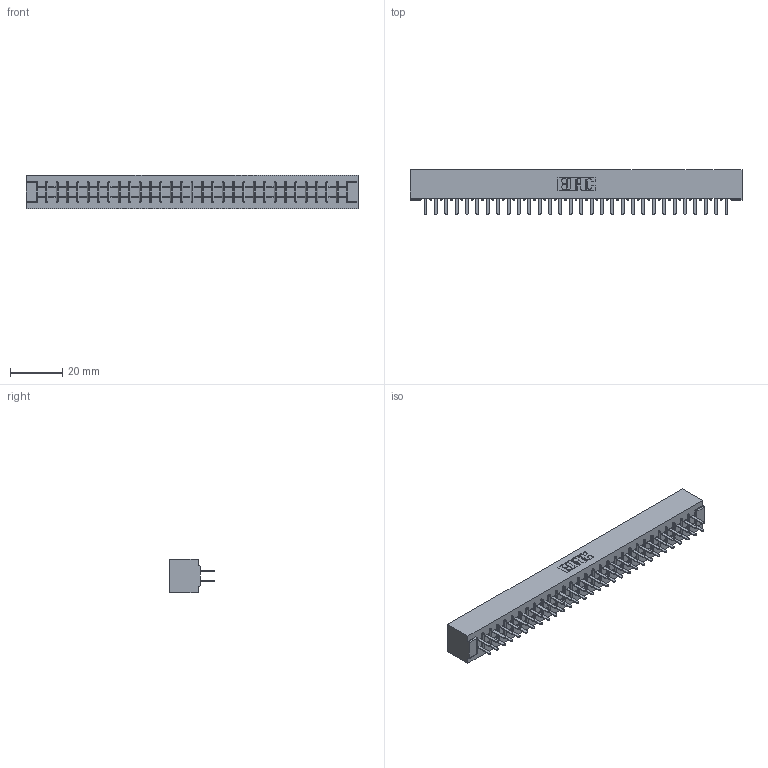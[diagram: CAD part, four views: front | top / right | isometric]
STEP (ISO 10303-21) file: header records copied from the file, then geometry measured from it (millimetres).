
FILE_DESCRIPTION (( 'STEP AP203' ), '1' );
FILE_NAME ('355-060-520-201.STEP', '2019-09-12T13:43:40', ( '' ), ( '' ), 'SwSTEP 2.0', 'SolidWorks 2016', '' );
FILE_SCHEMA (( 'CONFIG_CONTROL_DESIGN' ));
Length unit declared in the file: inch
Products named in the file (3): 355-060-520-201; 305-290-001_520; 305 Part_No Mounting
Assembly tree (61 placements, depth 2):
  355-060-520-201
    305 Part_No Mounting
    305-290-001_520  x60
Bounding box: 126.75 x 17.09 x 12.7 mm (x, y, z)
Volume: 13626.1 mm3; surface area: 17520.6 mm2
Topology: 61 solids, 61 shells, 2868 faces, 8182 edges, 5292 vertices
Faces by surface type: plane 1684, cylinder 1064, sphere 120
Entity records: 33545 total; most frequent: CARTESIAN_POINT 5548, ORIENTED_EDGE 5504, DIRECTION 5374, EDGE_CURVE 2752, LINE 2218, VECTOR 2218, VERTEX_POINT 1752, AXIS2_PLACEMENT_3D 1578
